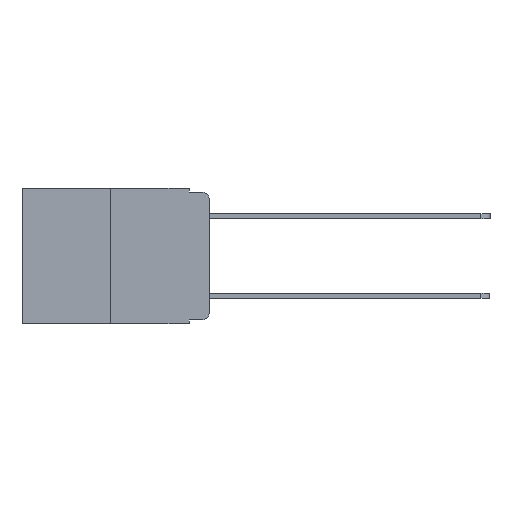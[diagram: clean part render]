
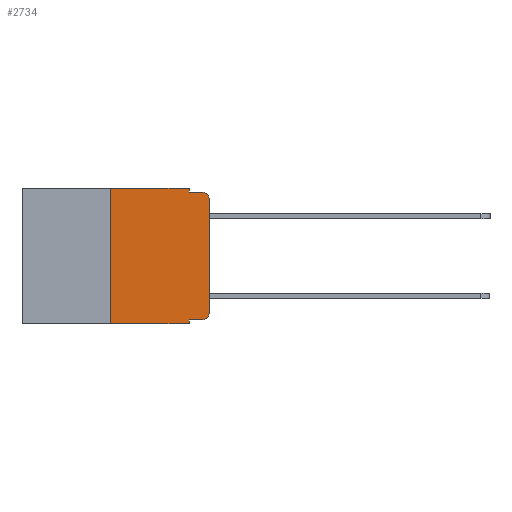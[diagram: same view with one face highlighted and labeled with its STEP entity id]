
A CAD part, left-side view. The second image highlights one B-rep face of the part: STEP entity #2734.
In plain terms, the highlighted planar face has unit normal (-1, 0, 0).
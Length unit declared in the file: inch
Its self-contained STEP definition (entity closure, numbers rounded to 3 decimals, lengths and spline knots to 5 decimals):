
#244 = EDGE_CURVE ( 'NONE', #10652, #1596, #12690, .T. ) ;
#520 = VECTOR ( 'NONE', #11997, 39.37008 ) ;
#897 = CARTESIAN_POINT ( 'NONE',  ( 0., 0.051, 0. ) ) ;
#1057 = CARTESIAN_POINT ( 'NONE',  ( 0., 0.02, -0.01 ) ) ;
#1084 = EDGE_CURVE ( 'NONE', #1596, #1855, #12513, .T. ) ;
#1094 = ORIENTED_EDGE ( 'NONE', *, *, #9024, .F. ) ;
#1468 = CARTESIAN_POINT ( 'NONE',  ( 0., 0.051, -0.333 ) ) ;
#1472 = CARTESIAN_POINT ( 'NONE',  ( 0., 0.25, -0.343 ) ) ;
#1596 = VERTEX_POINT ( 'NONE', #7715 ) ;
#1599 = DIRECTION ( 'NONE',  ( 0., -1., 0. ) ) ;
#1855 = VERTEX_POINT ( 'NONE', #9485 ) ;
#2013 = CARTESIAN_POINT ( 'NONE',  ( 0., 0.051, 0. ) ) ;
#2126 = ORIENTED_EDGE ( 'NONE', *, *, #12749, .F. ) ;
#2130 = VERTEX_POINT ( 'NONE', #4059 ) ;
#2545 = LINE ( 'NONE', #897, #7809 ) ;
#2734 = ADVANCED_FACE ( 'NONE', ( #13098 ), #4919, .F. ) ;
#2815 = DIRECTION ( 'NONE',  ( 0., -1., 0. ) ) ;
#2841 = LINE ( 'NONE', #12130, #5109 ) ;
#2874 = VERTEX_POINT ( 'NONE', #1472 ) ;
#3042 = ORIENTED_EDGE ( 'NONE', *, *, #8741, .F. ) ;
#3060 = DIRECTION ( 'NONE',  ( -1., 0., 0. ) ) ;
#3107 = CARTESIAN_POINT ( 'NONE',  ( 0., 0.051, -0.343 ) ) ;
#3132 = EDGE_CURVE ( 'NONE', #2874, #4821, #11510, .T. ) ;
#3242 = EDGE_LOOP ( 'NONE', ( #6337, #6918, #5676, #1094, #3042, #9903, #7805, #2126, #11136, #6187 ) ) ;
#3392 = VERTEX_POINT ( 'NONE', #1057 ) ;
#3413 = AXIS2_PLACEMENT_3D ( 'NONE', #3613, #3060, #10085 ) ;
#3613 = CARTESIAN_POINT ( 'NONE',  ( 0., 0.02, -0.313 ) ) ;
#3862 = AXIS2_PLACEMENT_3D ( 'NONE', #7586, #7564, #7539 ) ;
#4059 = CARTESIAN_POINT ( 'NONE',  ( 0., 0., -0.03 ) ) ;
#4064 = CARTESIAN_POINT ( 'NONE',  ( 0., 0.051, 0. ) ) ;
#4206 = DIRECTION ( 'NONE',  ( 1., 0., 0. ) ) ;
#4356 = VERTEX_POINT ( 'NONE', #5268 ) ;
#4409 = DIRECTION ( 'NONE',  ( 0., 0., 1. ) ) ;
#4412 = DIRECTION ( 'NONE',  ( 0., 0., -1. ) ) ;
#4821 = VERTEX_POINT ( 'NONE', #3107 ) ;
#4919 = PLANE ( 'NONE',  #8876 ) ;
#5109 = VECTOR ( 'NONE', #4409, 39.37008 ) ;
#5268 = CARTESIAN_POINT ( 'NONE',  ( 0., 0.051, -0.01 ) ) ;
#5385 = DIRECTION ( 'NONE',  ( 0., -1., 0. ) ) ;
#5676 = ORIENTED_EDGE ( 'NONE', *, *, #9654, .F. ) ;
#6187 = ORIENTED_EDGE ( 'NONE', *, *, #1084, .T. ) ;
#6249 = CARTESIAN_POINT ( 'NONE',  ( 0., 0.473, 0. ) ) ;
#6265 = CIRCLE ( 'NONE', #3862, 0.02 ) ;
#6283 = LINE ( 'NONE', #8880, #8553 ) ;
#6337 = ORIENTED_EDGE ( 'NONE', *, *, #8417, .T. ) ;
#6416 = LINE ( 'NONE', #2013, #520 ) ;
#6539 = CARTESIAN_POINT ( 'NONE',  ( 0., 0.25, 0. ) ) ;
#6918 = ORIENTED_EDGE ( 'NONE', *, *, #7144, .T. ) ;
#7144 = EDGE_CURVE ( 'NONE', #2130, #3392, #6265, .T. ) ;
#7174 = VECTOR ( 'NONE', #2815, 39.37008 ) ;
#7539 = DIRECTION ( 'NONE',  ( 0., 0., -1. ) ) ;
#7564 = DIRECTION ( 'NONE',  ( -1., 0., 0. ) ) ;
#7586 = CARTESIAN_POINT ( 'NONE',  ( 0., 0.02, -0.03 ) ) ;
#7715 = CARTESIAN_POINT ( 'NONE',  ( 0., 0.02, -0.333 ) ) ;
#7805 = ORIENTED_EDGE ( 'NONE', *, *, #3132, .T. ) ;
#7809 = VECTOR ( 'NONE', #10166, 39.37008 ) ;
#8017 = CARTESIAN_POINT ( 'NONE',  ( 0., 0.473, -0.343 ) ) ;
#8164 = VERTEX_POINT ( 'NONE', #4064 ) ;
#8295 = DIRECTION ( 'NONE',  ( 0., -1., 0. ) ) ;
#8417 = EDGE_CURVE ( 'NONE', #1855, #2130, #12603, .T. ) ;
#8445 = CARTESIAN_POINT ( 'NONE',  ( 0., 0., 0. ) ) ;
#8553 = VECTOR ( 'NONE', #1599, 39.37008 ) ;
#8741 = EDGE_CURVE ( 'NONE', #11538, #8164, #6283, .T. ) ;
#8876 = AXIS2_PLACEMENT_3D ( 'NONE', #6249, #4206, #4412 ) ;
#8880 = CARTESIAN_POINT ( 'NONE',  ( 0., 0.473, 0. ) ) ;
#9024 = EDGE_CURVE ( 'NONE', #8164, #4356, #2545, .T. ) ;
#9485 = CARTESIAN_POINT ( 'NONE',  ( 0., 0., -0.313 ) ) ;
#9654 = EDGE_CURVE ( 'NONE', #4356, #3392, #13143, .T. ) ;
#9869 = VECTOR ( 'NONE', #12107, 39.37008 ) ;
#9903 = ORIENTED_EDGE ( 'NONE', *, *, #12122, .F. ) ;
#10085 = DIRECTION ( 'NONE',  ( 0., 0., -1. ) ) ;
#10166 = DIRECTION ( 'NONE',  ( 0., 0., -1. ) ) ;
#10652 = VERTEX_POINT ( 'NONE', #1468 ) ;
#10700 = VECTOR ( 'NONE', #8295, 39.37008 ) ;
#11062 = CARTESIAN_POINT ( 'NONE',  ( 0., 0.051, -0.01 ) ) ;
#11136 = ORIENTED_EDGE ( 'NONE', *, *, #244, .T. ) ;
#11161 = CARTESIAN_POINT ( 'NONE',  ( 0., 0.051, -0.333 ) ) ;
#11221 = VECTOR ( 'NONE', #5385, 39.37008 ) ;
#11510 = LINE ( 'NONE', #8017, #11221 ) ;
#11538 = VERTEX_POINT ( 'NONE', #6539 ) ;
#11997 = DIRECTION ( 'NONE',  ( 0., 0., -1. ) ) ;
#12107 = DIRECTION ( 'NONE',  ( 0., 0., 1. ) ) ;
#12122 = EDGE_CURVE ( 'NONE', #2874, #11538, #2841, .T. ) ;
#12130 = CARTESIAN_POINT ( 'NONE',  ( 0., 0.25, 0. ) ) ;
#12513 = CIRCLE ( 'NONE', #3413, 0.02 ) ;
#12603 = LINE ( 'NONE', #8445, #9869 ) ;
#12690 = LINE ( 'NONE', #11161, #7174 ) ;
#12749 = EDGE_CURVE ( 'NONE', #10652, #4821, #6416, .T. ) ;
#13098 = FACE_OUTER_BOUND ( 'NONE', #3242, .T. ) ;
#13143 = LINE ( 'NONE', #11062, #10700 ) ;
